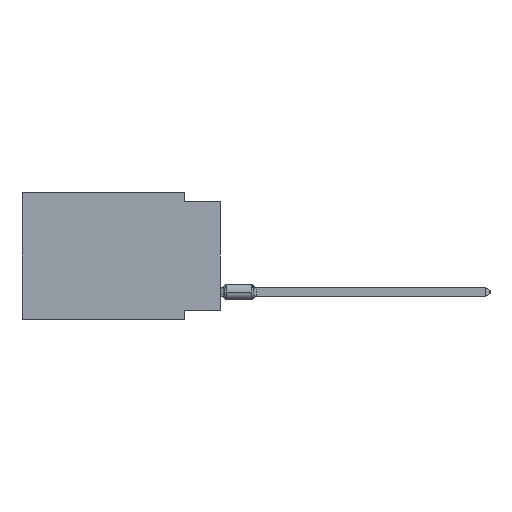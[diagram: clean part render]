
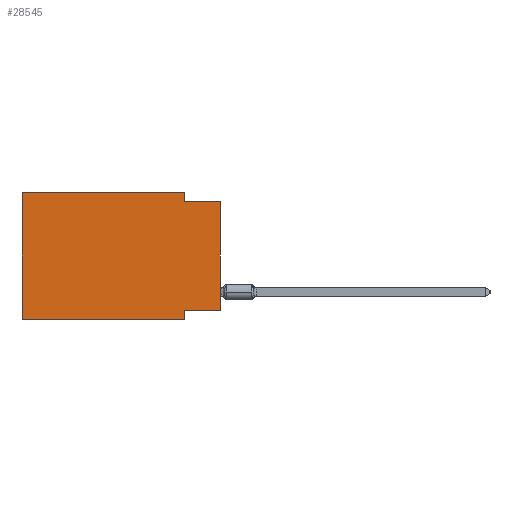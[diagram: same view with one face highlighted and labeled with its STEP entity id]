
A CAD part, left-side view. The second image highlights one B-rep face of the part: STEP entity #28545.
In plain terms, the highlighted planar face has unit normal (-1, 0, 0).
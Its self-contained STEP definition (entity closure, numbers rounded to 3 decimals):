
#37 = VERTEX_POINT ( 'NONE', #6964 ) ;
#1374 = ORIENTED_EDGE ( 'NONE', *, *, #5824, .F. ) ;
#1465 = EDGE_CURVE ( 'NONE', #24375, #48022, #43292, .T. ) ;
#1885 = DIRECTION ( 'NONE',  ( 0., 0., -1. ) ) ;
#2358 = FACE_OUTER_BOUND ( 'NONE', #6971, .T. ) ;
#2650 = CARTESIAN_POINT ( 'NONE',  ( 0., 13.97, 0. ) ) ;
#3718 = CARTESIAN_POINT ( 'NONE',  ( 0., 13.97, 0. ) ) ;
#4222 = ORIENTED_EDGE ( 'NONE', *, *, #5274, .T. ) ;
#5274 = EDGE_CURVE ( 'NONE', #10593, #22848, #44118, .T. ) ;
#5316 = CARTESIAN_POINT ( 'NONE',  ( 0., 2.54, 0. ) ) ;
#5613 = CARTESIAN_POINT ( 'NONE',  ( 0., 13.97, 0. ) ) ;
#5824 = EDGE_CURVE ( 'NONE', #20492, #22848, #45304, .T. ) ;
#6620 = LINE ( 'NONE', #10329, #45193 ) ;
#6964 = CARTESIAN_POINT ( 'NONE',  ( 0., 0., -8.255 ) ) ;
#6971 = EDGE_LOOP ( 'NONE', ( #43924, #30658, #14217, #40818, #47352, #4222, #1374, #43809 ) ) ;
#8657 = VECTOR ( 'NONE', #12323, 1000. ) ;
#9346 = DIRECTION ( 'NONE',  ( 0., 0., -1. ) ) ;
#10213 = LINE ( 'NONE', #32043, #20798 ) ;
#10329 = CARTESIAN_POINT ( 'NONE',  ( 0., 0., -8.255 ) ) ;
#10593 = VERTEX_POINT ( 'NONE', #10679 ) ;
#10679 = CARTESIAN_POINT ( 'NONE',  ( 0., 13.97, -8.89 ) ) ;
#11756 = VECTOR ( 'NONE', #44619, 1000. ) ;
#12323 = DIRECTION ( 'NONE',  ( 0., 0., 1. ) ) ;
#13220 = DIRECTION ( 'NONE',  ( 0., -1., 0. ) ) ;
#13829 = DIRECTION ( 'NONE',  ( 0., 1., 0. ) ) ;
#14217 = ORIENTED_EDGE ( 'NONE', *, *, #1465, .F. ) ;
#14916 = LINE ( 'NONE', #30027, #30095 ) ;
#15074 = EDGE_CURVE ( 'NONE', #10593, #22884, #31140, .T. ) ;
#16729 = EDGE_CURVE ( 'NONE', #37, #32744, #14916, .T. ) ;
#17792 = CARTESIAN_POINT ( 'NONE',  ( 0., 2.54, -8.89 ) ) ;
#18786 = CARTESIAN_POINT ( 'NONE',  ( 0., 2.54, -8.89 ) ) ;
#18859 = DIRECTION ( 'NONE',  ( 0., -1., 0. ) ) ;
#18941 = VECTOR ( 'NONE', #44790, 1000. ) ;
#19065 = VECTOR ( 'NONE', #9346, 1000. ) ;
#19363 = DIRECTION ( 'NONE',  ( 0., 0., 1. ) ) ;
#20442 = CARTESIAN_POINT ( 'NONE',  ( 0., 13.97, -8.89 ) ) ;
#20492 = VERTEX_POINT ( 'NONE', #36790 ) ;
#20798 = VECTOR ( 'NONE', #13220, 1000. ) ;
#22206 = CARTESIAN_POINT ( 'NONE',  ( 0., 2.54, -0.635 ) ) ;
#22848 = VERTEX_POINT ( 'NONE', #17792 ) ;
#22884 = VERTEX_POINT ( 'NONE', #2650 ) ;
#24375 = VERTEX_POINT ( 'NONE', #5316 ) ;
#28545 = ADVANCED_FACE ( 'NONE', ( #2358 ), #43991, .F. ) ;
#30027 = CARTESIAN_POINT ( 'NONE',  ( 0., 0., 0. ) ) ;
#30095 = VECTOR ( 'NONE', #19363, 1000. ) ;
#30658 = ORIENTED_EDGE ( 'NONE', *, *, #39997, .F. ) ;
#31140 = LINE ( 'NONE', #46259, #8657 ) ;
#31909 = CARTESIAN_POINT ( 'NONE',  ( 0., 2.54, 0. ) ) ;
#32043 = CARTESIAN_POINT ( 'NONE',  ( 0., 0., -0.635 ) ) ;
#32709 = CARTESIAN_POINT ( 'NONE',  ( 0., 0., -0.635 ) ) ;
#32744 = VERTEX_POINT ( 'NONE', #32709 ) ;
#34120 = EDGE_CURVE ( 'NONE', #22884, #24375, #37434, .T. ) ;
#35846 = DIRECTION ( 'NONE',  ( 1., 0., 0. ) ) ;
#36790 = CARTESIAN_POINT ( 'NONE',  ( 0., 2.54, -8.255 ) ) ;
#37434 = LINE ( 'NONE', #3718, #48180 ) ;
#39997 = EDGE_CURVE ( 'NONE', #48022, #32744, #10213, .T. ) ;
#40818 = ORIENTED_EDGE ( 'NONE', *, *, #34120, .F. ) ;
#41133 = AXIS2_PLACEMENT_3D ( 'NONE', #5613, #35846, #1885 ) ;
#43292 = LINE ( 'NONE', #31909, #19065 ) ;
#43809 = ORIENTED_EDGE ( 'NONE', *, *, #44275, .F. ) ;
#43924 = ORIENTED_EDGE ( 'NONE', *, *, #16729, .T. ) ;
#43991 = PLANE ( 'NONE',  #41133 ) ;
#44118 = LINE ( 'NONE', #20442, #11756 ) ;
#44275 = EDGE_CURVE ( 'NONE', #37, #20492, #6620, .T. ) ;
#44619 = DIRECTION ( 'NONE',  ( 0., -1., 0. ) ) ;
#44790 = DIRECTION ( 'NONE',  ( 0., 0., -1. ) ) ;
#45193 = VECTOR ( 'NONE', #13829, 1000. ) ;
#45304 = LINE ( 'NONE', #18786, #18941 ) ;
#46259 = CARTESIAN_POINT ( 'NONE',  ( 0., 13.97, 0. ) ) ;
#47352 = ORIENTED_EDGE ( 'NONE', *, *, #15074, .F. ) ;
#48022 = VERTEX_POINT ( 'NONE', #22206 ) ;
#48180 = VECTOR ( 'NONE', #18859, 1000. ) ;
